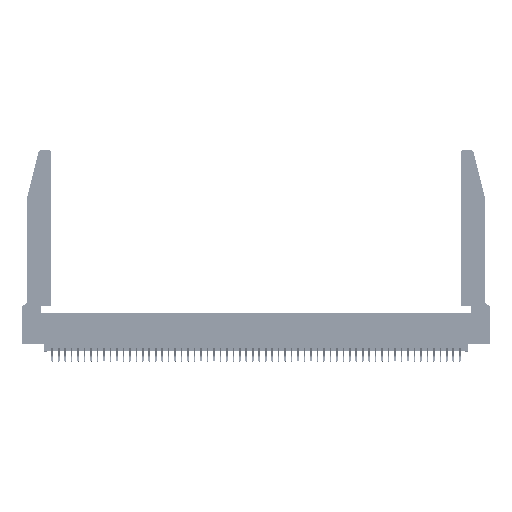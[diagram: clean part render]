
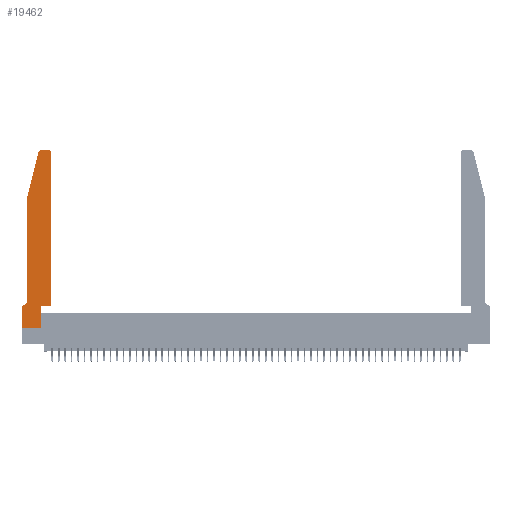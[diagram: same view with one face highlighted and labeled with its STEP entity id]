
A CAD part, top view. The second image highlights one B-rep face of the part: STEP entity #19462.
In plain terms, the highlighted planar face has unit normal (0, 0, 1).
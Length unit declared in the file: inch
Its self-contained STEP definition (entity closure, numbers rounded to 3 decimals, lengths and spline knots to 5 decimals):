
#290 = CARTESIAN_POINT ( 'NONE',  ( 0.284, 2.75, 0.37 ) ) ;
#651 = VERTEX_POINT ( 'NONE', #7310 ) ;
#1262 = ORIENTED_EDGE ( 'NONE', *, *, #13900, .T. ) ;
#1350 = VERTEX_POINT ( 'NONE', #15660 ) ;
#1813 = CARTESIAN_POINT ( 'NONE',  ( 0.0755, 2., 0.37 ) ) ;
#2163 = EDGE_CURVE ( 'NONE', #8322, #8373, #49290, .T. ) ;
#3661 = EDGE_CURVE ( 'NONE', #41456, #10854, #35951, .T. ) ;
#3898 = EDGE_CURVE ( 'NONE', #651, #48280, #4211, .T. ) ;
#4211 = LINE ( 'NONE', #27104, #45965 ) ;
#7290 = DIRECTION ( 'NONE',  ( 0., 1., 0. ) ) ;
#7310 = CARTESIAN_POINT ( 'NONE',  ( 0.4205, 2.75, 0.37 ) ) ;
#7987 = AXIS2_PLACEMENT_3D ( 'NONE', #10063, #38272, #14146 ) ;
#8322 = VERTEX_POINT ( 'NONE', #21435 ) ;
#8373 = VERTEX_POINT ( 'NONE', #45845 ) ;
#9108 = AXIS2_PLACEMENT_3D ( 'NONE', #10350, #38562, #14430 ) ;
#9524 = EDGE_CURVE ( 'NONE', #30394, #1350, #14263, .T. ) ;
#10063 = CARTESIAN_POINT ( 'NONE',  ( 0.4205, 2.72, 0.37 ) ) ;
#10350 = CARTESIAN_POINT ( 'NONE',  ( 0.0055, 0.42, 0.37 ) ) ;
#10854 = VERTEX_POINT ( 'NONE', #48271 ) ;
#11140 = VERTEX_POINT ( 'NONE', #13580 ) ;
#12365 = ORIENTED_EDGE ( 'NONE', *, *, #45187, .T. ) ;
#13580 = CARTESIAN_POINT ( 'NONE',  ( 0.2865, 0., 0.37 ) ) ;
#13799 = ORIENTED_EDGE ( 'NONE', *, *, #38287, .T. ) ;
#13900 = EDGE_CURVE ( 'NONE', #47140, #8322, #28389, .T. ) ;
#14146 = DIRECTION ( 'NONE',  ( 1., 0., 0. ) ) ;
#14263 = LINE ( 'NONE', #36459, #34404 ) ;
#14430 = DIRECTION ( 'NONE',  ( -1., 0., 0. ) ) ;
#15660 = CARTESIAN_POINT ( 'NONE',  ( 0.4505, 0.35, 0.37 ) ) ;
#15814 = VECTOR ( 'NONE', #49627, 39.37008 ) ;
#16516 = DIRECTION ( 'NONE',  ( 0., 0., 1. ) ) ;
#16995 = AXIS2_PLACEMENT_3D ( 'NONE', #40594, #16516, #44641 ) ;
#17274 = ORIENTED_EDGE ( 'NONE', *, *, #3898, .T. ) ;
#18291 = VERTEX_POINT ( 'NONE', #30426 ) ;
#18383 = DIRECTION ( 'NONE',  ( 0., 1., 0. ) ) ;
#18723 = LINE ( 'NONE', #27587, #31908 ) ;
#18821 = CARTESIAN_POINT ( 'NONE',  ( 0.2865, 0.35, 0.37 ) ) ;
#18984 = VECTOR ( 'NONE', #26204, 39.37008 ) ;
#19462 = ADVANCED_FACE ( 'NONE', ( #25898 ), #35496, .T. ) ;
#19519 = CARTESIAN_POINT ( 'NONE',  ( 0.0055, 0.35, 0.37 ) ) ;
#19537 = DIRECTION ( 'NONE',  ( 1., 0., 0. ) ) ;
#20147 = CIRCLE ( 'NONE', #16995, 0.03 ) ;
#20741 = EDGE_CURVE ( 'NONE', #11140, #30394, #32777, .T. ) ;
#20852 = VECTOR ( 'NONE', #7290, 39.37008 ) ;
#21232 = ORIENTED_EDGE ( 'NONE', *, *, #20741, .T. ) ;
#21435 = CARTESIAN_POINT ( 'NONE',  ( 0.0755, 2., 0.37 ) ) ;
#21703 = CARTESIAN_POINT ( 'NONE',  ( 0.0755, 0.35, 0.37 ) ) ;
#25557 = LINE ( 'NONE', #39793, #36267 ) ;
#25898 = FACE_OUTER_BOUND ( 'NONE', #36523, .T. ) ;
#26204 = DIRECTION ( 'NONE',  ( -0.239, -0.971, 0. ) ) ;
#27104 = CARTESIAN_POINT ( 'NONE',  ( 0.2605, 2.75, 0.37 ) ) ;
#27352 = ORIENTED_EDGE ( 'NONE', *, *, #2163, .T. ) ;
#27587 = CARTESIAN_POINT ( 'NONE',  ( 0., 0., 0.37 ) ) ;
#28389 = LINE ( 'NONE', #1813, #18984 ) ;
#28530 = DIRECTION ( 'NONE',  ( 1., 0., 0. ) ) ;
#28781 = DIRECTION ( 'NONE',  ( 0., -1., 0. ) ) ;
#29145 = CARTESIAN_POINT ( 'NONE',  ( 0.4505, 2.72, 0.37 ) ) ;
#29293 = CARTESIAN_POINT ( 'NONE',  ( 0.0755, 2., 0.37 ) ) ;
#29452 = VECTOR ( 'NONE', #18383, 39.37008 ) ;
#29554 = CARTESIAN_POINT ( 'NONE',  ( 0.25487, 2.72718, 0.37 ) ) ;
#30032 = ORIENTED_EDGE ( 'NONE', *, *, #3661, .T. ) ;
#30394 = VERTEX_POINT ( 'NONE', #18821 ) ;
#30426 = CARTESIAN_POINT ( 'NONE',  ( 0., 0., 0.37 ) ) ;
#31169 = DIRECTION ( 'NONE',  ( -1., 0., 0. ) ) ;
#31305 = ORIENTED_EDGE ( 'NONE', *, *, #36270, .T. ) ;
#31908 = VECTOR ( 'NONE', #51638, 39.37008 ) ;
#31948 = ORIENTED_EDGE ( 'NONE', *, *, #33553, .T. ) ;
#32777 = LINE ( 'NONE', #35569, #20852 ) ;
#33553 = EDGE_CURVE ( 'NONE', #37378, #651, #46856, .T. ) ;
#34404 = VECTOR ( 'NONE', #28530, 39.37008 ) ;
#35011 = AXIS2_PLACEMENT_3D ( 'NONE', #39543, #43560, #19537 ) ;
#35496 = PLANE ( 'NONE',  #35011 ) ;
#35569 = CARTESIAN_POINT ( 'NONE',  ( 0.2865, 0.35, 0.37 ) ) ;
#35951 = LINE ( 'NONE', #21703, #15814 ) ;
#36267 = VECTOR ( 'NONE', #43836, 39.37008 ) ;
#36270 = EDGE_CURVE ( 'NONE', #8373, #41456, #37233, .T. ) ;
#36459 = CARTESIAN_POINT ( 'NONE',  ( 0.4505, 0.35, 0.37 ) ) ;
#36523 = EDGE_LOOP ( 'NONE', ( #17274, #47544, #1262, #27352, #31305, #30032, #38841, #12365, #21232, #46514, #13799, #31948 ) ) ;
#37233 = CIRCLE ( 'NONE', #9108, 0.07 ) ;
#37276 = EDGE_CURVE ( 'NONE', #48280, #47140, #20147, .T. ) ;
#37378 = VERTEX_POINT ( 'NONE', #29145 ) ;
#38272 = DIRECTION ( 'NONE',  ( 0., 0., 1. ) ) ;
#38287 = EDGE_CURVE ( 'NONE', #1350, #37378, #49559, .T. ) ;
#38562 = DIRECTION ( 'NONE',  ( 0., 0., -1. ) ) ;
#38634 = VECTOR ( 'NONE', #28781, 39.37008 ) ;
#38841 = ORIENTED_EDGE ( 'NONE', *, *, #43964, .T. ) ;
#39543 = CARTESIAN_POINT ( 'NONE',  ( 0., 0.35, 0.37 ) ) ;
#39793 = CARTESIAN_POINT ( 'NONE',  ( 0., 0., 0.37 ) ) ;
#40594 = CARTESIAN_POINT ( 'NONE',  ( 0.284, 2.72, 0.37 ) ) ;
#41456 = VERTEX_POINT ( 'NONE', #19519 ) ;
#43560 = DIRECTION ( 'NONE',  ( 0., 0., 1. ) ) ;
#43836 = DIRECTION ( 'NONE',  ( 1., 0., 0. ) ) ;
#43964 = EDGE_CURVE ( 'NONE', #10854, #18291, #18723, .T. ) ;
#44641 = DIRECTION ( 'NONE',  ( 1., 0., 0. ) ) ;
#45187 = EDGE_CURVE ( 'NONE', #18291, #11140, #25557, .T. ) ;
#45845 = CARTESIAN_POINT ( 'NONE',  ( 0.0755, 0.42, 0.37 ) ) ;
#45965 = VECTOR ( 'NONE', #31169, 39.37008 ) ;
#46485 = CARTESIAN_POINT ( 'NONE',  ( 0.4505, 0.35, 0.37 ) ) ;
#46514 = ORIENTED_EDGE ( 'NONE', *, *, #9524, .T. ) ;
#46856 = CIRCLE ( 'NONE', #7987, 0.03 ) ;
#47140 = VERTEX_POINT ( 'NONE', #29554 ) ;
#47544 = ORIENTED_EDGE ( 'NONE', *, *, #37276, .T. ) ;
#48271 = CARTESIAN_POINT ( 'NONE',  ( 0., 0.35, 0.37 ) ) ;
#48280 = VERTEX_POINT ( 'NONE', #290 ) ;
#49290 = LINE ( 'NONE', #29293, #38634 ) ;
#49559 = LINE ( 'NONE', #46485, #29452 ) ;
#49627 = DIRECTION ( 'NONE',  ( -1., 0., 0. ) ) ;
#51638 = DIRECTION ( 'NONE',  ( 0., -1., 0. ) ) ;
